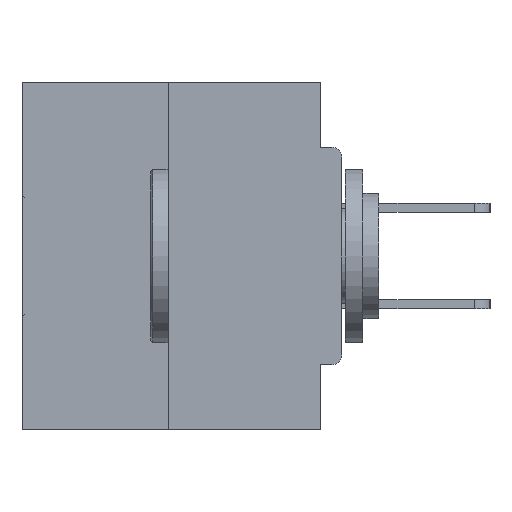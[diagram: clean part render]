
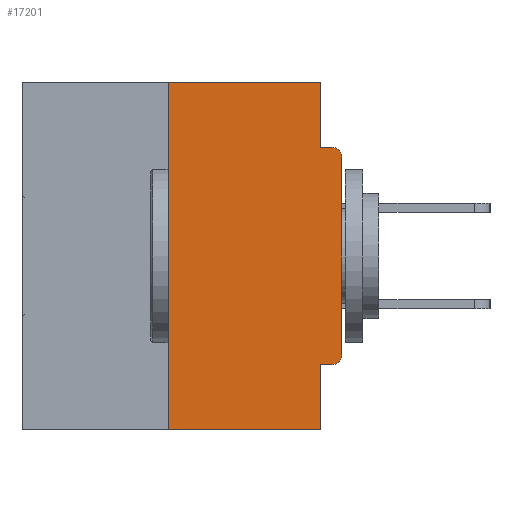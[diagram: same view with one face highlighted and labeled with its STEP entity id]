
A CAD part, left-side view. The second image highlights one B-rep face of the part: STEP entity #17201.
In plain terms, the highlighted planar face has unit normal (-1, 0, 0).
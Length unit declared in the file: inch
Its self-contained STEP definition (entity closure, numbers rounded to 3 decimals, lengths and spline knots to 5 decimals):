
#1123 = EDGE_CURVE ( 'NONE', #26949, #25923, #26277, .T. ) ;
#1378 = FACE_OUTER_BOUND ( 'NONE', #4337, .T. ) ;
#1769 = DIRECTION ( 'NONE',  ( -1., 0., 0. ) ) ;
#1969 = EDGE_CURVE ( 'NONE', #38395, #20474, #10574, .T. ) ;
#3022 = VECTOR ( 'NONE', #21521, 39.37008 ) ;
#3068 = EDGE_CURVE ( 'NONE', #31400, #38948, #13388, .T. ) ;
#3082 = DIRECTION ( 'NONE',  ( 0., 0., -1. ) ) ;
#3152 = CARTESIAN_POINT ( 'NONE',  ( 0., 0.031, -0.5 ) ) ;
#3835 = CARTESIAN_POINT ( 'NONE',  ( 0., 0., -0.4065 ) ) ;
#4166 = DIRECTION ( 'NONE',  ( 0., 0., -1. ) ) ;
#4337 = EDGE_LOOP ( 'NONE', ( #18639, #26516, #11269, #13377, #35874, #40566, #20242, #37796, #9811, #28861 ) ) ;
#5534 = VERTEX_POINT ( 'NONE', #40599 ) ;
#5920 = EDGE_CURVE ( 'NONE', #17332, #13397, #9126, .T. ) ;
#7560 = CARTESIAN_POINT ( 'NONE',  ( 0., 0.015, -0.0935 ) ) ;
#8901 = DIRECTION ( 'NONE',  ( 0., 0., 1. ) ) ;
#9126 = LINE ( 'NONE', #26714, #15439 ) ;
#9811 = ORIENTED_EDGE ( 'NONE', *, *, #29999, .F. ) ;
#10574 = LINE ( 'NONE', #21457, #34559 ) ;
#11269 = ORIENTED_EDGE ( 'NONE', *, *, #37532, .T. ) ;
#11321 = LINE ( 'NONE', #12390, #35311 ) ;
#11533 = DIRECTION ( 'NONE',  ( 0., 0., -1. ) ) ;
#12390 = CARTESIAN_POINT ( 'NONE',  ( 0., 0., -0.0935 ) ) ;
#13078 = CARTESIAN_POINT ( 'NONE',  ( 0., 0.46, 0. ) ) ;
#13377 = ORIENTED_EDGE ( 'NONE', *, *, #15824, .F. ) ;
#13388 = CIRCLE ( 'NONE', #18333, 0.015 ) ;
#13397 = VERTEX_POINT ( 'NONE', #28281 ) ;
#14072 = CARTESIAN_POINT ( 'NONE',  ( 0., 0.25, 0. ) ) ;
#15159 = DIRECTION ( 'NONE',  ( 0., -1., 0. ) ) ;
#15439 = VECTOR ( 'NONE', #11533, 39.37008 ) ;
#15824 = EDGE_CURVE ( 'NONE', #5534, #30138, #21143, .T. ) ;
#17201 = ADVANCED_FACE ( 'NONE', ( #1378 ), #22664, .F. ) ;
#17332 = VERTEX_POINT ( 'NONE', #20020 ) ;
#18333 = AXIS2_PLACEMENT_3D ( 'NONE', #27732, #40241, #3082 ) ;
#18639 = ORIENTED_EDGE ( 'NONE', *, *, #21731, .F. ) ;
#19641 = DIRECTION ( 'NONE',  ( 1., 0., 0. ) ) ;
#19703 = DIRECTION ( 'NONE',  ( 0., 1., 0. ) ) ;
#19926 = CARTESIAN_POINT ( 'NONE',  ( 0., 0.46, -0.5 ) ) ;
#20020 = CARTESIAN_POINT ( 'NONE',  ( 0., 0.031, 0. ) ) ;
#20242 = ORIENTED_EDGE ( 'NONE', *, *, #28573, .T. ) ;
#20444 = CARTESIAN_POINT ( 'NONE',  ( 0., 0., 0. ) ) ;
#20474 = VERTEX_POINT ( 'NONE', #14072 ) ;
#20581 = CARTESIAN_POINT ( 'NONE',  ( 0., 0.25, -0.5 ) ) ;
#21143 = LINE ( 'NONE', #3152, #3022 ) ;
#21457 = CARTESIAN_POINT ( 'NONE',  ( 0., 0.25, 0. ) ) ;
#21521 = DIRECTION ( 'NONE',  ( 0., 0., -1. ) ) ;
#21566 = CARTESIAN_POINT ( 'NONE',  ( 0., 0.46, 0. ) ) ;
#21731 = EDGE_CURVE ( 'NONE', #20474, #17332, #37385, .T. ) ;
#21985 = CARTESIAN_POINT ( 'NONE',  ( 0., 0.015, -0.4065 ) ) ;
#22127 = CARTESIAN_POINT ( 'NONE',  ( 0., 0., -0.1085 ) ) ;
#22664 = PLANE ( 'NONE',  #30381 ) ;
#23281 = VECTOR ( 'NONE', #19703, 39.37008 ) ;
#23460 = LINE ( 'NONE', #20444, #31211 ) ;
#24436 = VECTOR ( 'NONE', #38587, 39.37008 ) ;
#25923 = VERTEX_POINT ( 'NONE', #7560 ) ;
#26277 = CIRCLE ( 'NONE', #39033, 0.015 ) ;
#26516 = ORIENTED_EDGE ( 'NONE', *, *, #1969, .F. ) ;
#26714 = CARTESIAN_POINT ( 'NONE',  ( 0., 0.031, 0. ) ) ;
#26859 = LINE ( 'NONE', #19926, #24436 ) ;
#26949 = VERTEX_POINT ( 'NONE', #22127 ) ;
#27732 = CARTESIAN_POINT ( 'NONE',  ( 0., 0.015, -0.3915 ) ) ;
#28120 = LINE ( 'NONE', #3835, #23281 ) ;
#28281 = CARTESIAN_POINT ( 'NONE',  ( 0., 0.031, -0.0935 ) ) ;
#28573 = EDGE_CURVE ( 'NONE', #38948, #26949, #23460, .T. ) ;
#28861 = ORIENTED_EDGE ( 'NONE', *, *, #5920, .F. ) ;
#29999 = EDGE_CURVE ( 'NONE', #13397, #25923, #11321, .T. ) ;
#30138 = VERTEX_POINT ( 'NONE', #34694 ) ;
#30381 = AXIS2_PLACEMENT_3D ( 'NONE', #13078, #19641, #4166 ) ;
#30448 = DIRECTION ( 'NONE',  ( 0., -1., 0. ) ) ;
#31211 = VECTOR ( 'NONE', #33298, 39.37008 ) ;
#31400 = VERTEX_POINT ( 'NONE', #21985 ) ;
#33287 = CARTESIAN_POINT ( 'NONE',  ( 0., 0.015, -0.1085 ) ) ;
#33298 = DIRECTION ( 'NONE',  ( 0., 0., 1. ) ) ;
#34559 = VECTOR ( 'NONE', #8901, 39.37008 ) ;
#34694 = CARTESIAN_POINT ( 'NONE',  ( 0., 0.031, -0.5 ) ) ;
#35311 = VECTOR ( 'NONE', #15159, 39.37008 ) ;
#35874 = ORIENTED_EDGE ( 'NONE', *, *, #39816, .F. ) ;
#36398 = VECTOR ( 'NONE', #30448, 39.37008 ) ;
#37385 = LINE ( 'NONE', #21566, #36398 ) ;
#37532 = EDGE_CURVE ( 'NONE', #38395, #30138, #26859, .T. ) ;
#37796 = ORIENTED_EDGE ( 'NONE', *, *, #1123, .T. ) ;
#38395 = VERTEX_POINT ( 'NONE', #20581 ) ;
#38587 = DIRECTION ( 'NONE',  ( 0., -1., 0. ) ) ;
#38948 = VERTEX_POINT ( 'NONE', #39585 ) ;
#39033 = AXIS2_PLACEMENT_3D ( 'NONE', #33287, #1769, #39622 ) ;
#39585 = CARTESIAN_POINT ( 'NONE',  ( 0., 0., -0.3915 ) ) ;
#39622 = DIRECTION ( 'NONE',  ( 0., 0., -1. ) ) ;
#39816 = EDGE_CURVE ( 'NONE', #31400, #5534, #28120, .T. ) ;
#40241 = DIRECTION ( 'NONE',  ( -1., 0., 0. ) ) ;
#40566 = ORIENTED_EDGE ( 'NONE', *, *, #3068, .T. ) ;
#40599 = CARTESIAN_POINT ( 'NONE',  ( 0., 0.031, -0.4065 ) ) ;
